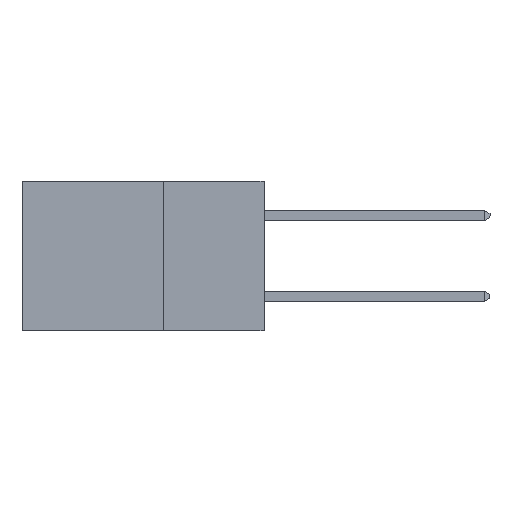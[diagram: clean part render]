
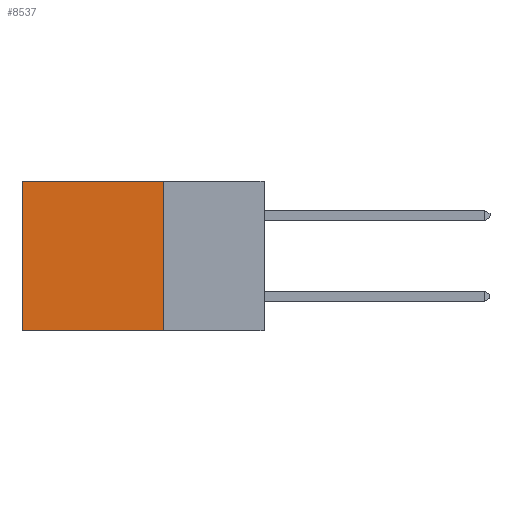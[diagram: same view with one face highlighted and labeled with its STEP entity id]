
A CAD part, left-side view. The second image highlights one B-rep face of the part: STEP entity #8537.
In plain terms, the highlighted planar face has unit normal (-1, 0, 0).
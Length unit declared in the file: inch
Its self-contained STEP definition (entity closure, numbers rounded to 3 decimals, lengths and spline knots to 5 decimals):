
#1175 = CARTESIAN_POINT ( 'NONE',  ( 0.298, 0.25, -0.37 ) ) ;
#1672 = CARTESIAN_POINT ( 'NONE',  ( 0.298, 0.25, 0. ) ) ;
#1714 = CARTESIAN_POINT ( 'NONE',  ( 0.298, 0.25, 0. ) ) ;
#1910 = VERTEX_POINT ( 'NONE', #6238 ) ;
#1985 = VERTEX_POINT ( 'NONE', #1175 ) ;
#2090 = AXIS2_PLACEMENT_3D ( 'NONE', #1714, #10409, #3873 ) ;
#2291 = VERTEX_POINT ( 'NONE', #2687 ) ;
#2409 = EDGE_CURVE ( 'NONE', #11398, #1910, #6780, .T. ) ;
#2617 = ORIENTED_EDGE ( 'NONE', *, *, #8153, .T. ) ;
#2687 = CARTESIAN_POINT ( 'NONE',  ( 0.298, 0.25, 0. ) ) ;
#2752 = DIRECTION ( 'NONE',  ( 0., 1., 0. ) ) ;
#2795 = PLANE ( 'NONE',  #2090 ) ;
#2889 = CARTESIAN_POINT ( 'NONE',  ( 0.298, 0.25, 0. ) ) ;
#3046 = DIRECTION ( 'NONE',  ( 0., 1., 0. ) ) ;
#3873 = DIRECTION ( 'NONE',  ( 0., 0., -1. ) ) ;
#5345 = EDGE_LOOP ( 'NONE', ( #9637, #7097, #7442, #2617 ) ) ;
#6238 = CARTESIAN_POINT ( 'NONE',  ( 0.298, 0.6, -0.37 ) ) ;
#6634 = DIRECTION ( 'NONE',  ( 0., 0., -1. ) ) ;
#6780 = LINE ( 'NONE', #7364, #9339 ) ;
#7097 = ORIENTED_EDGE ( 'NONE', *, *, #9894, .F. ) ;
#7364 = CARTESIAN_POINT ( 'NONE',  ( 0.298, 0.6, 0. ) ) ;
#7442 = ORIENTED_EDGE ( 'NONE', *, *, #12042, .F. ) ;
#8153 = EDGE_CURVE ( 'NONE', #2291, #11398, #12814, .T. ) ;
#8354 = DIRECTION ( 'NONE',  ( 0., 0., -1. ) ) ;
#8537 = ADVANCED_FACE ( 'NONE', ( #10452 ), #2795, .F. ) ;
#9208 = VECTOR ( 'NONE', #8354, 39.37008 ) ;
#9339 = VECTOR ( 'NONE', #6634, 39.37008 ) ;
#9417 = LINE ( 'NONE', #9592, #12136 ) ;
#9419 = CARTESIAN_POINT ( 'NONE',  ( 0.298, 0.6, 0. ) ) ;
#9592 = CARTESIAN_POINT ( 'NONE',  ( 0.298, 0.25, -0.37 ) ) ;
#9637 = ORIENTED_EDGE ( 'NONE', *, *, #2409, .T. ) ;
#9894 = EDGE_CURVE ( 'NONE', #1985, #1910, #9417, .T. ) ;
#10409 = DIRECTION ( 'NONE',  ( 1., 0., 0. ) ) ;
#10452 = FACE_OUTER_BOUND ( 'NONE', #5345, .T. ) ;
#11398 = VERTEX_POINT ( 'NONE', #9419 ) ;
#12042 = EDGE_CURVE ( 'NONE', #2291, #1985, #12246, .T. ) ;
#12136 = VECTOR ( 'NONE', #3046, 39.37008 ) ;
#12186 = VECTOR ( 'NONE', #2752, 39.37008 ) ;
#12246 = LINE ( 'NONE', #2889, #9208 ) ;
#12814 = LINE ( 'NONE', #1672, #12186 ) ;
